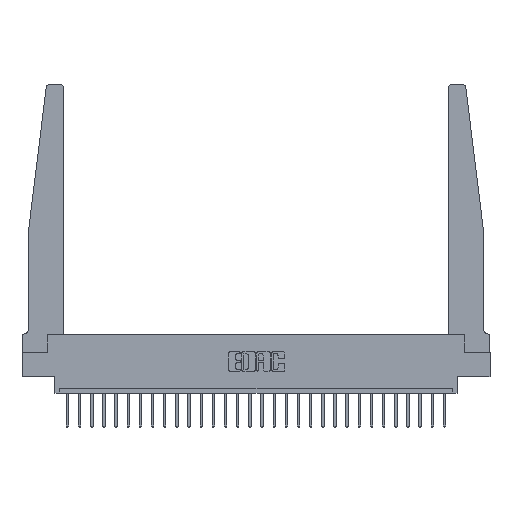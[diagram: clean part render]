
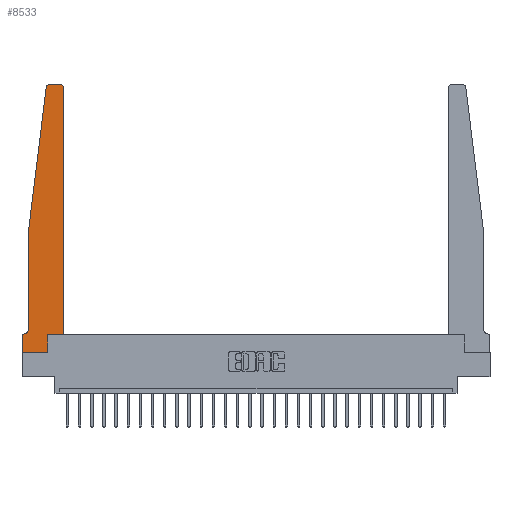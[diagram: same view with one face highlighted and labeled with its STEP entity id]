
A CAD part, top view. The second image highlights one B-rep face of the part: STEP entity #8533.
In plain terms, the highlighted planar face has unit normal (0, 0, 1).
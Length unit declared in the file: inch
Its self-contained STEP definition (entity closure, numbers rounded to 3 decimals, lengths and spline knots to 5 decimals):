
#93 = CARTESIAN_POINT ( 'NONE',  ( 0.065, 0.2375, 0.37 ) ) ;
#229 = DIRECTION ( 'NONE',  ( 0., 0., 1. ) ) ;
#532 = EDGE_CURVE ( 'NONE', #7371, #15858, #24108, .T. ) ;
#586 = DIRECTION ( 'NONE',  ( 1., 0., 0. ) ) ;
#948 = DIRECTION ( 'NONE',  ( -1., 0., 0. ) ) ;
#1014 = LINE ( 'NONE', #17197, #2267 ) ;
#1209 = EDGE_CURVE ( 'NONE', #3385, #1765, #1014, .T. ) ;
#1765 = VERTEX_POINT ( 'NONE', #13549 ) ;
#1791 = LINE ( 'NONE', #8938, #4671 ) ;
#2216 = DIRECTION ( 'NONE',  ( 1., 0., 0. ) ) ;
#2267 = VECTOR ( 'NONE', #13291, 39.37008 ) ;
#2820 = AXIS2_PLACEMENT_3D ( 'NONE', #7301, #10963, #948 ) ;
#3369 = CIRCLE ( 'NONE', #24540, 0.03 ) ;
#3385 = VERTEX_POINT ( 'NONE', #16055 ) ;
#3480 = ORIENTED_EDGE ( 'NONE', *, *, #10857, .T. ) ;
#3921 = DIRECTION ( 'NONE',  ( 0., 1., 0. ) ) ;
#4114 = VERTEX_POINT ( 'NONE', #20110 ) ;
#4256 = VECTOR ( 'NONE', #19212, 39.37008 ) ;
#4641 = VECTOR ( 'NONE', #8555, 39.37008 ) ;
#4651 = ORIENTED_EDGE ( 'NONE', *, *, #20910, .T. ) ;
#4671 = VECTOR ( 'NONE', #16763, 39.37008 ) ;
#5080 = CARTESIAN_POINT ( 'NONE',  ( 0.015, 0.1875, 0.37 ) ) ;
#5491 = CIRCLE ( 'NONE', #2820, 0.05 ) ;
#5715 = VERTEX_POINT ( 'NONE', #7021 ) ;
#6484 = ORIENTED_EDGE ( 'NONE', *, *, #25026, .T. ) ;
#7021 = CARTESIAN_POINT ( 'NONE',  ( 0.2605, 0., 0.37 ) ) ;
#7271 = LINE ( 'NONE', #20167, #24944 ) ;
#7301 = CARTESIAN_POINT ( 'NONE',  ( 0.015, 0.2375, 0.37 ) ) ;
#7371 = VERTEX_POINT ( 'NONE', #17231 ) ;
#7372 = AXIS2_PLACEMENT_3D ( 'NONE', #10251, #229, #586 ) ;
#7736 = ORIENTED_EDGE ( 'NONE', *, *, #24131, .T. ) ;
#7815 = DIRECTION ( 'NONE',  ( 0., 0., 1. ) ) ;
#8533 = ADVANCED_FACE ( 'NONE', ( #10704 ), #22315, .T. ) ;
#8555 = DIRECTION ( 'NONE',  ( 0., -1., 0. ) ) ;
#8726 = CIRCLE ( 'NONE', #14873, 0.03 ) ;
#8830 = CARTESIAN_POINT ( 'NONE',  ( 0.065, 1.25, 0.37 ) ) ;
#8938 = CARTESIAN_POINT ( 'NONE',  ( 0.065, 0.1875, 0.37 ) ) ;
#9187 = CARTESIAN_POINT ( 'NONE',  ( 0.425, 0.18, 0.37 ) ) ;
#9404 = LINE ( 'NONE', #10820, #24547 ) ;
#9981 = VERTEX_POINT ( 'NONE', #13855 ) ;
#10209 = ORIENTED_EDGE ( 'NONE', *, *, #532, .T. ) ;
#10251 = CARTESIAN_POINT ( 'NONE',  ( 0., 0.1875, 0.37 ) ) ;
#10704 = FACE_OUTER_BOUND ( 'NONE', #14192, .T. ) ;
#10820 = CARTESIAN_POINT ( 'NONE',  ( 0., 0., 0.37 ) ) ;
#10857 = EDGE_CURVE ( 'NONE', #1765, #18886, #15031, .T. ) ;
#10931 = DIRECTION ( 'NONE',  ( 0., 1., 0. ) ) ;
#10963 = DIRECTION ( 'NONE',  ( 0., 0., -1. ) ) ;
#11208 = LINE ( 'NONE', #14058, #4641 ) ;
#11436 = ORIENTED_EDGE ( 'NONE', *, *, #25461, .T. ) ;
#11464 = VERTEX_POINT ( 'NONE', #5080 ) ;
#12538 = ORIENTED_EDGE ( 'NONE', *, *, #1209, .T. ) ;
#12606 = VERTEX_POINT ( 'NONE', #21071 ) ;
#12701 = VECTOR ( 'NONE', #10931, 39.37008 ) ;
#12720 = ORIENTED_EDGE ( 'NONE', *, *, #17678, .T. ) ;
#13291 = DIRECTION ( 'NONE',  ( -0.122, -0.992, 0. ) ) ;
#13452 = VECTOR ( 'NONE', #25147, 39.37008 ) ;
#13549 = CARTESIAN_POINT ( 'NONE',  ( 0.065, 1.25, 0.37 ) ) ;
#13855 = CARTESIAN_POINT ( 'NONE',  ( 0., 0.1875, 0.37 ) ) ;
#14058 = CARTESIAN_POINT ( 'NONE',  ( 0., 0., 0.37 ) ) ;
#14192 = EDGE_LOOP ( 'NONE', ( #11436, #7736, #12538, #3480, #4651, #21313, #20077, #12720, #23740, #10209, #20014, #6484 ) ) ;
#14231 = DIRECTION ( 'NONE',  ( 0., 0., 1. ) ) ;
#14873 = AXIS2_PLACEMENT_3D ( 'NONE', #16059, #7815, #20118 ) ;
#14875 = DIRECTION ( 'NONE',  ( 1., 0., 0. ) ) ;
#15031 = LINE ( 'NONE', #8830, #13452 ) ;
#15858 = VERTEX_POINT ( 'NONE', #21519 ) ;
#15871 = LINE ( 'NONE', #9187, #12701 ) ;
#16055 = CARTESIAN_POINT ( 'NONE',  ( 0.24675, 2.72367, 0.37 ) ) ;
#16059 = CARTESIAN_POINT ( 'NONE',  ( 0.27653, 2.72, 0.37 ) ) ;
#16524 = EDGE_CURVE ( 'NONE', #5715, #7371, #7271, .T. ) ;
#16763 = DIRECTION ( 'NONE',  ( -1., 0., 0. ) ) ;
#16937 = DIRECTION ( 'NONE',  ( -1., 0., 0. ) ) ;
#17182 = CARTESIAN_POINT ( 'NONE',  ( 0.425, 0.18, 0.37 ) ) ;
#17197 = CARTESIAN_POINT ( 'NONE',  ( 0.065, 1.25, 0.37 ) ) ;
#17231 = CARTESIAN_POINT ( 'NONE',  ( 0.2605, 0.18, 0.37 ) ) ;
#17678 = EDGE_CURVE ( 'NONE', #21078, #5715, #9404, .T. ) ;
#18262 = CARTESIAN_POINT ( 'NONE',  ( 0.25, 2.75, 0.37 ) ) ;
#18886 = VERTEX_POINT ( 'NONE', #93 ) ;
#19059 = VERTEX_POINT ( 'NONE', #24310 ) ;
#19212 = DIRECTION ( 'NONE',  ( 1., 0., 0. ) ) ;
#19997 = LINE ( 'NONE', #18262, #26039 ) ;
#20014 = ORIENTED_EDGE ( 'NONE', *, *, #25677, .T. ) ;
#20077 = ORIENTED_EDGE ( 'NONE', *, *, #24496, .T. ) ;
#20110 = CARTESIAN_POINT ( 'NONE',  ( 0.27653, 2.75, 0.37 ) ) ;
#20118 = DIRECTION ( 'NONE',  ( 1., 0., 0. ) ) ;
#20167 = CARTESIAN_POINT ( 'NONE',  ( 0.2605, 0.18, 0.37 ) ) ;
#20408 = CARTESIAN_POINT ( 'NONE',  ( 0., 0., 0.37 ) ) ;
#20910 = EDGE_CURVE ( 'NONE', #18886, #11464, #5491, .T. ) ;
#21071 = CARTESIAN_POINT ( 'NONE',  ( 0.395, 2.75, 0.37 ) ) ;
#21078 = VERTEX_POINT ( 'NONE', #20408 ) ;
#21313 = ORIENTED_EDGE ( 'NONE', *, *, #24303, .T. ) ;
#21519 = CARTESIAN_POINT ( 'NONE',  ( 0.425, 0.18, 0.37 ) ) ;
#22315 = PLANE ( 'NONE',  #7372 ) ;
#22360 = CARTESIAN_POINT ( 'NONE',  ( 0.395, 2.72, 0.37 ) ) ;
#23740 = ORIENTED_EDGE ( 'NONE', *, *, #16524, .T. ) ;
#24108 = LINE ( 'NONE', #17182, #4256 ) ;
#24131 = EDGE_CURVE ( 'NONE', #4114, #3385, #8726, .T. ) ;
#24303 = EDGE_CURVE ( 'NONE', #11464, #9981, #1791, .T. ) ;
#24310 = CARTESIAN_POINT ( 'NONE',  ( 0.425, 2.72, 0.37 ) ) ;
#24496 = EDGE_CURVE ( 'NONE', #9981, #21078, #11208, .T. ) ;
#24540 = AXIS2_PLACEMENT_3D ( 'NONE', #22360, #14231, #2216 ) ;
#24547 = VECTOR ( 'NONE', #14875, 39.37008 ) ;
#24944 = VECTOR ( 'NONE', #3921, 39.37008 ) ;
#25026 = EDGE_CURVE ( 'NONE', #19059, #12606, #3369, .T. ) ;
#25147 = DIRECTION ( 'NONE',  ( 0., -1., 0. ) ) ;
#25461 = EDGE_CURVE ( 'NONE', #12606, #4114, #19997, .T. ) ;
#25677 = EDGE_CURVE ( 'NONE', #15858, #19059, #15871, .T. ) ;
#26039 = VECTOR ( 'NONE', #16937, 39.37008 ) ;
